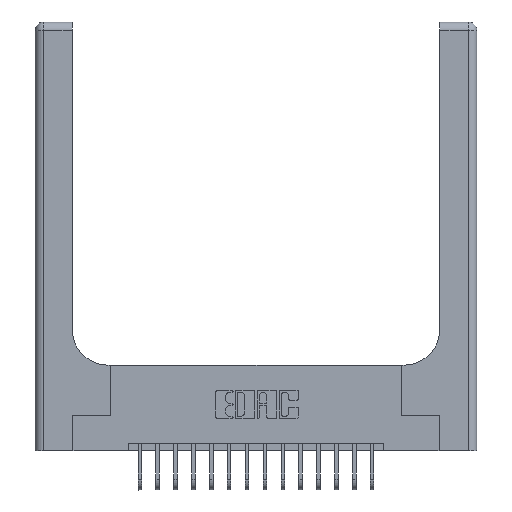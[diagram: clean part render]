
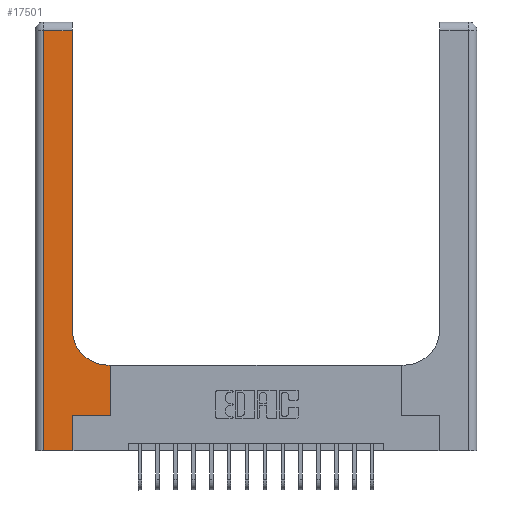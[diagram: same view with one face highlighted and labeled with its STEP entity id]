
A CAD part, top view. The second image highlights one B-rep face of the part: STEP entity #17501.
In plain terms, the highlighted planar face has unit normal (0, 0, 1).
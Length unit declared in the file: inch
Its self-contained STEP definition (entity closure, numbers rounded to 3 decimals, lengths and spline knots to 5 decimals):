
#63 = LINE ( 'NONE', #12988, #6999 ) ;
#191 = CARTESIAN_POINT ( 'NONE',  ( 0.06, 3., 0.37 ) ) ;
#228 = VERTEX_POINT ( 'NONE', #10970 ) ;
#407 = DIRECTION ( 'NONE',  ( 0., 1., 0. ) ) ;
#680 = LINE ( 'NONE', #12932, #11225 ) ;
#847 = CARTESIAN_POINT ( 'NONE',  ( 0.528, 0.25, 0.37 ) ) ;
#1591 = DIRECTION ( 'NONE',  ( 0., -1., 0. ) ) ;
#1637 = CARTESIAN_POINT ( 'NONE',  ( 0.06, 0., 0.37 ) ) ;
#2256 = DIRECTION ( 'NONE',  ( 0., 1., 0. ) ) ;
#2572 = EDGE_LOOP ( 'NONE', ( #9713, #7391, #11770, #16213, #16200, #17122, #4259, #2586, #14636 ) ) ;
#2586 = ORIENTED_EDGE ( 'NONE', *, *, #6768, .T. ) ;
#2789 = PLANE ( 'NONE',  #4711 ) ;
#3368 = CARTESIAN_POINT ( 'NONE',  ( 0.51, 0.6, 0.37 ) ) ;
#3373 = LINE ( 'NONE', #10927, #17024 ) ;
#3455 = LINE ( 'NONE', #13923, #9470 ) ;
#4259 = ORIENTED_EDGE ( 'NONE', *, *, #15219, .T. ) ;
#4493 = EDGE_CURVE ( 'NONE', #12627, #5760, #3373, .T. ) ;
#4567 = LINE ( 'NONE', #9115, #8247 ) ;
#4711 = AXIS2_PLACEMENT_3D ( 'NONE', #13718, #5549, #15101 ) ;
#5015 = DIRECTION ( 'NONE',  ( 1., 0., 0. ) ) ;
#5332 = VERTEX_POINT ( 'NONE', #3368 ) ;
#5549 = DIRECTION ( 'NONE',  ( 0., 0., -1. ) ) ;
#5760 = VERTEX_POINT ( 'NONE', #9882 ) ;
#6129 = DIRECTION ( 'NONE',  ( -1., 0., 0. ) ) ;
#6189 = VERTEX_POINT ( 'NONE', #9695 ) ;
#6615 = DIRECTION ( 'NONE',  ( 0., 0., -1. ) ) ;
#6768 = EDGE_CURVE ( 'NONE', #6189, #5332, #680, .T. ) ;
#6841 = CARTESIAN_POINT ( 'NONE',  ( 0.265, 0.25, 0.37 ) ) ;
#6999 = VECTOR ( 'NONE', #9013, 39.37008 ) ;
#7353 = CARTESIAN_POINT ( 'NONE',  ( 0.06, 2.94, 0.37 ) ) ;
#7391 = ORIENTED_EDGE ( 'NONE', *, *, #16795, .T. ) ;
#7619 = VECTOR ( 'NONE', #5015, 39.37008 ) ;
#8247 = VECTOR ( 'NONE', #17245, 39.37008 ) ;
#8597 = FACE_OUTER_BOUND ( 'NONE', #2572, .T. ) ;
#9013 = DIRECTION ( 'NONE',  ( 0., 1., 0. ) ) ;
#9115 = CARTESIAN_POINT ( 'NONE',  ( 0., 2.94, 0.37 ) ) ;
#9236 = EDGE_CURVE ( 'NONE', #13583, #12627, #3455, .T. ) ;
#9332 = LINE ( 'NONE', #191, #16131 ) ;
#9470 = VECTOR ( 'NONE', #407, 39.37008 ) ;
#9695 = CARTESIAN_POINT ( 'NONE',  ( 0.528, 0.6, 0.37 ) ) ;
#9713 = ORIENTED_EDGE ( 'NONE', *, *, #14179, .T. ) ;
#9882 = CARTESIAN_POINT ( 'NONE',  ( 0.528, 0.25, 0.37 ) ) ;
#9987 = LINE ( 'NONE', #847, #16786 ) ;
#10605 = VERTEX_POINT ( 'NONE', #10883 ) ;
#10883 = CARTESIAN_POINT ( 'NONE',  ( 0.26, 0.85, 0.37 ) ) ;
#10927 = CARTESIAN_POINT ( 'NONE',  ( 0.265, 0.25, 0.37 ) ) ;
#10970 = CARTESIAN_POINT ( 'NONE',  ( 0.26, 2.94, 0.37 ) ) ;
#11225 = VECTOR ( 'NONE', #6129, 39.37008 ) ;
#11770 = ORIENTED_EDGE ( 'NONE', *, *, #16025, .T. ) ;
#12176 = CIRCLE ( 'NONE', #14735, 0.25 ) ;
#12292 = DIRECTION ( 'NONE',  ( 1., 0., 0. ) ) ;
#12496 = EDGE_CURVE ( 'NONE', #5332, #10605, #12176, .T. ) ;
#12627 = VERTEX_POINT ( 'NONE', #6841 ) ;
#12932 = CARTESIAN_POINT ( 'NONE',  ( 0.26, 0.6, 0.37 ) ) ;
#12988 = CARTESIAN_POINT ( 'NONE',  ( 0.26, 3., 0.37 ) ) ;
#13220 = CARTESIAN_POINT ( 'NONE',  ( 0., 0., 0.37 ) ) ;
#13583 = VERTEX_POINT ( 'NONE', #15928 ) ;
#13718 = CARTESIAN_POINT ( 'NONE',  ( 0., 3., 0.37 ) ) ;
#13923 = CARTESIAN_POINT ( 'NONE',  ( 0.265, 0., 0.37 ) ) ;
#13946 = VERTEX_POINT ( 'NONE', #1637 ) ;
#14179 = EDGE_CURVE ( 'NONE', #10605, #228, #63, .T. ) ;
#14636 = ORIENTED_EDGE ( 'NONE', *, *, #12496, .T. ) ;
#14735 = AXIS2_PLACEMENT_3D ( 'NONE', #14773, #6615, #16138 ) ;
#14773 = CARTESIAN_POINT ( 'NONE',  ( 0.51, 0.85, 0.37 ) ) ;
#14855 = EDGE_CURVE ( 'NONE', #13946, #13583, #14861, .T. ) ;
#14861 = LINE ( 'NONE', #13220, #7619 ) ;
#15101 = DIRECTION ( 'NONE',  ( -1., 0., 0. ) ) ;
#15219 = EDGE_CURVE ( 'NONE', #5760, #6189, #9987, .T. ) ;
#15928 = CARTESIAN_POINT ( 'NONE',  ( 0.265, 0., 0.37 ) ) ;
#16025 = EDGE_CURVE ( 'NONE', #17602, #13946, #9332, .T. ) ;
#16131 = VECTOR ( 'NONE', #1591, 39.37008 ) ;
#16138 = DIRECTION ( 'NONE',  ( 1., 0., 0. ) ) ;
#16200 = ORIENTED_EDGE ( 'NONE', *, *, #9236, .T. ) ;
#16213 = ORIENTED_EDGE ( 'NONE', *, *, #14855, .T. ) ;
#16786 = VECTOR ( 'NONE', #2256, 39.37008 ) ;
#16795 = EDGE_CURVE ( 'NONE', #228, #17602, #4567, .T. ) ;
#17024 = VECTOR ( 'NONE', #12292, 39.37008 ) ;
#17122 = ORIENTED_EDGE ( 'NONE', *, *, #4493, .T. ) ;
#17245 = DIRECTION ( 'NONE',  ( -1., 0., 0. ) ) ;
#17501 = ADVANCED_FACE ( 'NONE', ( #8597 ), #2789, .F. ) ;
#17602 = VERTEX_POINT ( 'NONE', #7353 ) ;
